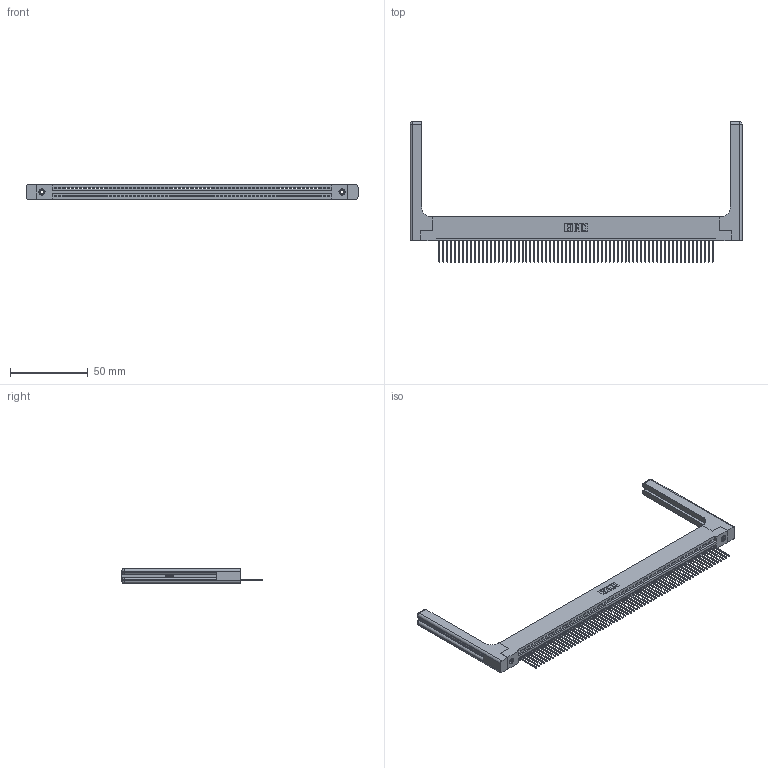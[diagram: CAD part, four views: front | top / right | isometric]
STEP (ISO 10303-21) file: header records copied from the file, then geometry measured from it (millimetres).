
FILE_DESCRIPTION (( 'STEP AP203' ), '1' );
FILE_NAME ('395-070-540-158.STEP', '2019-10-26T00:42:25', ( '' ), ( '' ), 'SwSTEP 2.0', 'SolidWorks 2016', '' );
FILE_SCHEMA (( 'CONFIG_CONTROL_DESIGN' ));
Length unit declared in the file: inch
Products named in the file (5): 345-250-001_345-250-001-102; 345 Part_Flush Mounting Lugs - 0.156 Dia-TH; 345-220-058_345-220-058; 345-292-001_345-293-140; 395-070-540-158
Assembly tree (75 placements, depth 2):
  395-070-540-158
    345 Part_Flush Mounting Lugs - 0.156 Dia-TH
    345-292-001_345-293-140  x70
    345-250-001_345-250-001-102  x2
    345-220-058_345-220-058  x2
Bounding box: 212.83 x 90.09 x 9.4 mm (x, y, z)
Volume: 29043.6 mm3; surface area: 33662.2 mm2
Topology: 75 solids, 75 shells, 4442 faces, 13327 edges, 8770 vertices
Faces by surface type: plane 3028, cylinder 1354, bspline 36, cone 12, sphere 8, torus 4
Entity records: 54114 total; most frequent: CARTESIAN_POINT 10343, ORIENTED_EDGE 9144, DIRECTION 7940, EDGE_CURVE 4572, LINE 4068, VECTOR 4068, VERTEX_POINT 3038, AXIS2_PLACEMENT_3D 1936
